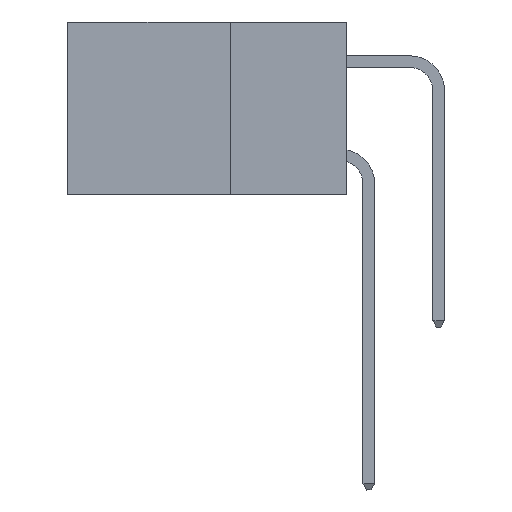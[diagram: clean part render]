
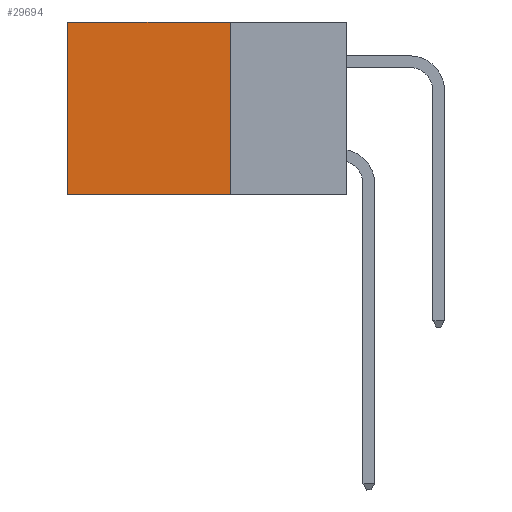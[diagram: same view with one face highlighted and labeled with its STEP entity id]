
A CAD part, left-side view. The second image highlights one B-rep face of the part: STEP entity #29694.
In plain terms, the highlighted planar face has unit normal (-1, 0, 0).
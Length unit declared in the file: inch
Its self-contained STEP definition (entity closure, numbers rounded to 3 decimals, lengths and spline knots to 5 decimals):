
#243 = CARTESIAN_POINT ( 'NONE',  ( 0.2875, 0.25, 0. ) ) ;
#272 = VECTOR ( 'NONE', #38780, 39.37008 ) ;
#2139 = CARTESIAN_POINT ( 'NONE',  ( 0.2875, 0.25, 0. ) ) ;
#2735 = LINE ( 'NONE', #13091, #15528 ) ;
#3824 = DIRECTION ( 'NONE',  ( 0., 1., 0. ) ) ;
#5222 = DIRECTION ( 'NONE',  ( 1., 0., 0. ) ) ;
#6386 = ORIENTED_EDGE ( 'NONE', *, *, #21379, .F. ) ;
#6570 = EDGE_CURVE ( 'NONE', #17524, #15764, #31442, .T. ) ;
#6737 = CARTESIAN_POINT ( 'NONE',  ( 0.2875, 0.25, -0.37 ) ) ;
#6955 = CARTESIAN_POINT ( 'NONE',  ( 0.2875, 0.6, 0. ) ) ;
#8149 = CARTESIAN_POINT ( 'NONE',  ( 0.2875, 0.6, 0. ) ) ;
#8910 = EDGE_LOOP ( 'NONE', ( #24401, #27044, #6386, #20650 ) ) ;
#12024 = VERTEX_POINT ( 'NONE', #36229 ) ;
#13091 = CARTESIAN_POINT ( 'NONE',  ( 0.2875, 0.25, 0. ) ) ;
#14214 = DIRECTION ( 'NONE',  ( 0., 0., -1. ) ) ;
#15184 = VECTOR ( 'NONE', #3824, 39.37008 ) ;
#15528 = VECTOR ( 'NONE', #38403, 39.37008 ) ;
#15764 = VERTEX_POINT ( 'NONE', #8149 ) ;
#17401 = LINE ( 'NONE', #6955, #26086 ) ;
#17524 = VERTEX_POINT ( 'NONE', #243 ) ;
#19522 = VERTEX_POINT ( 'NONE', #29773 ) ;
#20650 = ORIENTED_EDGE ( 'NONE', *, *, #6570, .T. ) ;
#21379 = EDGE_CURVE ( 'NONE', #17524, #12024, #2735, .T. ) ;
#22361 = EDGE_CURVE ( 'NONE', #15764, #19522, #17401, .T. ) ;
#23607 = CARTESIAN_POINT ( 'NONE',  ( 0.2875, 0.25, 0. ) ) ;
#24401 = ORIENTED_EDGE ( 'NONE', *, *, #22361, .T. ) ;
#25176 = EDGE_CURVE ( 'NONE', #12024, #19522, #32552, .T. ) ;
#26086 = VECTOR ( 'NONE', #27857, 39.37008 ) ;
#27044 = ORIENTED_EDGE ( 'NONE', *, *, #25176, .F. ) ;
#27857 = DIRECTION ( 'NONE',  ( 0., 0., -1. ) ) ;
#29694 = ADVANCED_FACE ( 'NONE', ( #30830 ), #30014, .F. ) ;
#29773 = CARTESIAN_POINT ( 'NONE',  ( 0.2875, 0.6, -0.37 ) ) ;
#30014 = PLANE ( 'NONE',  #39300 ) ;
#30830 = FACE_OUTER_BOUND ( 'NONE', #8910, .T. ) ;
#31442 = LINE ( 'NONE', #23607, #272 ) ;
#32552 = LINE ( 'NONE', #6737, #15184 ) ;
#36229 = CARTESIAN_POINT ( 'NONE',  ( 0.2875, 0.25, -0.37 ) ) ;
#38403 = DIRECTION ( 'NONE',  ( 0., 0., -1. ) ) ;
#38780 = DIRECTION ( 'NONE',  ( 0., 1., 0. ) ) ;
#39300 = AXIS2_PLACEMENT_3D ( 'NONE', #2139, #5222, #14214 ) ;
